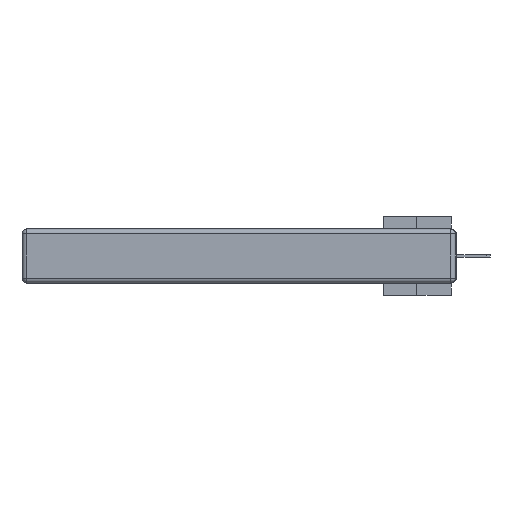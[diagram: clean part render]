
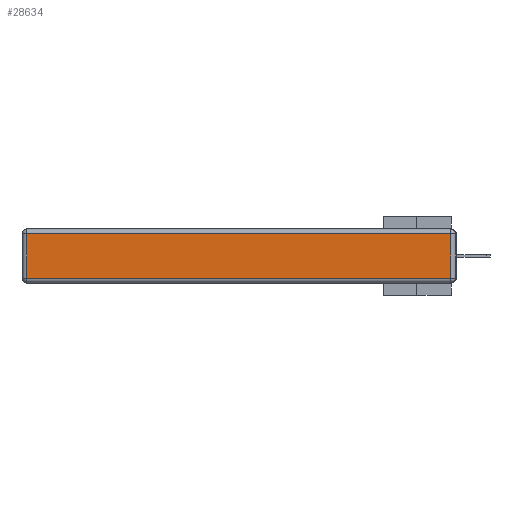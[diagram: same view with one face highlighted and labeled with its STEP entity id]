
A CAD part, left-side view. The second image highlights one B-rep face of the part: STEP entity #28634.
In plain terms, the highlighted planar face has unit normal (-1, 0, 0).
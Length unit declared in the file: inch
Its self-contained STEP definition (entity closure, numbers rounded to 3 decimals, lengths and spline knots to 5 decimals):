
#2803 = CARTESIAN_POINT ( 'NONE',  ( 0., 0., -0.313 ) ) ;
#2852 = EDGE_LOOP ( 'NONE', ( #17472, #33409, #22985, #15328 ) ) ;
#2891 = VERTEX_POINT ( 'NONE', #10062 ) ;
#4774 = EDGE_CURVE ( 'NONE', #2891, #5215, #8304, .T. ) ;
#4994 = CARTESIAN_POINT ( 'NONE',  ( 0., 2.75, -0.03 ) ) ;
#5041 = PLANE ( 'NONE',  #24011 ) ;
#5215 = VERTEX_POINT ( 'NONE', #32442 ) ;
#7804 = DIRECTION ( 'NONE',  ( 0., 0., 1. ) ) ;
#8304 = LINE ( 'NONE', #2803, #18474 ) ;
#8468 = DIRECTION ( 'NONE',  ( 0., -1., 0. ) ) ;
#8616 = DIRECTION ( 'NONE',  ( 0., 0., -1. ) ) ;
#9433 = VECTOR ( 'NONE', #23649, 39.37008 ) ;
#10062 = CARTESIAN_POINT ( 'NONE',  ( 0., 2.72, -0.313 ) ) ;
#10255 = CARTESIAN_POINT ( 'NONE',  ( 0., 0.03, -0.03 ) ) ;
#11336 = DIRECTION ( 'NONE',  ( 0., 0., 1. ) ) ;
#13039 = LINE ( 'NONE', #4994, #9433 ) ;
#15328 = ORIENTED_EDGE ( 'NONE', *, *, #19917, .T. ) ;
#15385 = EDGE_CURVE ( 'NONE', #5215, #25148, #16634, .T. ) ;
#15442 = VECTOR ( 'NONE', #11336, 39.37008 ) ;
#16634 = LINE ( 'NONE', #24859, #15442 ) ;
#17066 = CARTESIAN_POINT ( 'NONE',  ( 0., 0., -0.343 ) ) ;
#17472 = ORIENTED_EDGE ( 'NONE', *, *, #4774, .T. ) ;
#18474 = VECTOR ( 'NONE', #8468, 39.37008 ) ;
#19917 = EDGE_CURVE ( 'NONE', #33459, #2891, #24360, .T. ) ;
#20216 = EDGE_CURVE ( 'NONE', #25148, #33459, #13039, .T. ) ;
#22129 = CARTESIAN_POINT ( 'NONE',  ( 0., 2.72, -0.343 ) ) ;
#22985 = ORIENTED_EDGE ( 'NONE', *, *, #20216, .T. ) ;
#23649 = DIRECTION ( 'NONE',  ( 0., 1., 0. ) ) ;
#24011 = AXIS2_PLACEMENT_3D ( 'NONE', #17066, #26084, #7804 ) ;
#24360 = LINE ( 'NONE', #22129, #26882 ) ;
#24611 = CARTESIAN_POINT ( 'NONE',  ( 0., 2.72, -0.03 ) ) ;
#24859 = CARTESIAN_POINT ( 'NONE',  ( 0., 0.03, -0.343 ) ) ;
#25148 = VERTEX_POINT ( 'NONE', #10255 ) ;
#26084 = DIRECTION ( 'NONE',  ( -1., 0., 0. ) ) ;
#26882 = VECTOR ( 'NONE', #8616, 39.37008 ) ;
#28511 = FACE_OUTER_BOUND ( 'NONE', #2852, .T. ) ;
#28634 = ADVANCED_FACE ( 'NONE', ( #28511 ), #5041, .T. ) ;
#32442 = CARTESIAN_POINT ( 'NONE',  ( 0., 0.03, -0.313 ) ) ;
#33409 = ORIENTED_EDGE ( 'NONE', *, *, #15385, .T. ) ;
#33459 = VERTEX_POINT ( 'NONE', #24611 ) ;
